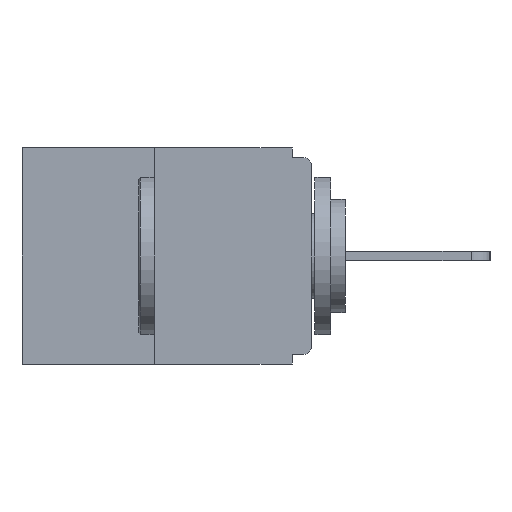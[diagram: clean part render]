
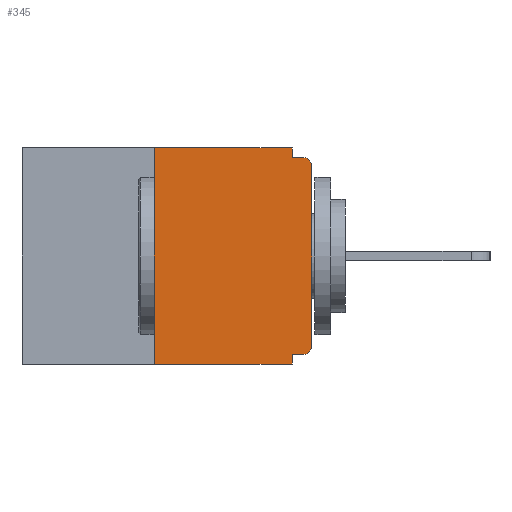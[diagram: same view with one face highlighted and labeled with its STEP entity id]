
A CAD part, left-side view. The second image highlights one B-rep face of the part: STEP entity #345.
In plain terms, the highlighted planar face has unit normal (-1, 0, 0).
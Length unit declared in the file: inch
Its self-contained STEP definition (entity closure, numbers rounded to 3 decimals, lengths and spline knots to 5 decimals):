
#185 = DIRECTION ( 'NONE',  ( -1., 0., 0. ) ) ;
#345 = ADVANCED_FACE ( 'NONE', ( #2129 ), #19526, .F. ) ;
#494 = VECTOR ( 'NONE', #15554, 39.37008 ) ;
#844 = DIRECTION ( 'NONE',  ( 0., 0., -1. ) ) ;
#1202 = ORIENTED_EDGE ( 'NONE', *, *, #11485, .F. ) ;
#1237 = CIRCLE ( 'NONE', #6461, 0.015 ) ;
#1445 = EDGE_CURVE ( 'NONE', #11963, #7149, #10571, .T. ) ;
#1454 = CIRCLE ( 'NONE', #1816, 0.015 ) ;
#1697 = CARTESIAN_POINT ( 'NONE',  ( 0., 0.015, -0.015 ) ) ;
#1816 = AXIS2_PLACEMENT_3D ( 'NONE', #4488, #185, #16967 ) ;
#1875 = CARTESIAN_POINT ( 'NONE',  ( 0., 0.25, 0. ) ) ;
#2006 = VECTOR ( 'NONE', #2769, 39.37008 ) ;
#2129 = FACE_OUTER_BOUND ( 'NONE', #8937, .T. ) ;
#2533 = VECTOR ( 'NONE', #11294, 39.37008 ) ;
#2769 = DIRECTION ( 'NONE',  ( 0., -1., 0. ) ) ;
#3111 = AXIS2_PLACEMENT_3D ( 'NONE', #14575, #17868, #8278 ) ;
#3160 = VECTOR ( 'NONE', #8622, 39.37008 ) ;
#3869 = DIRECTION ( 'NONE',  ( 0., -1., 0. ) ) ;
#3902 = VERTEX_POINT ( 'NONE', #8051 ) ;
#3907 = LINE ( 'NONE', #19870, #3160 ) ;
#3956 = ORIENTED_EDGE ( 'NONE', *, *, #17641, .F. ) ;
#4488 = CARTESIAN_POINT ( 'NONE',  ( 0., 0.015, -0.03 ) ) ;
#4532 = EDGE_CURVE ( 'NONE', #10491, #7149, #1454, .T. ) ;
#4659 = VECTOR ( 'NONE', #15467, 39.37008 ) ;
#4820 = EDGE_CURVE ( 'NONE', #3902, #16959, #5487, .T. ) ;
#4845 = ORIENTED_EDGE ( 'NONE', *, *, #18654, .F. ) ;
#5487 = LINE ( 'NONE', #10337, #8335 ) ;
#5598 = ORIENTED_EDGE ( 'NONE', *, *, #19945, .T. ) ;
#5983 = ORIENTED_EDGE ( 'NONE', *, *, #17176, .F. ) ;
#6461 = AXIS2_PLACEMENT_3D ( 'NONE', #16472, #16691, #844 ) ;
#6522 = LINE ( 'NONE', #12842, #2533 ) ;
#6594 = LINE ( 'NONE', #6694, #9418 ) ;
#6694 = CARTESIAN_POINT ( 'NONE',  ( 0., 0.46, 0. ) ) ;
#7149 = VERTEX_POINT ( 'NONE', #1697 ) ;
#7938 = CARTESIAN_POINT ( 'NONE',  ( 0., 0., -0.313 ) ) ;
#8051 = CARTESIAN_POINT ( 'NONE',  ( 0., 0.25, -0.343 ) ) ;
#8278 = DIRECTION ( 'NONE',  ( 0., 0., -1. ) ) ;
#8335 = VECTOR ( 'NONE', #3869, 39.37008 ) ;
#8622 = DIRECTION ( 'NONE',  ( 0., 0., -1. ) ) ;
#8937 = EDGE_LOOP ( 'NONE', ( #3956, #15534, #14204, #1202, #5983, #5598, #11415, #13940, #19472, #4845 ) ) ;
#9338 = EDGE_CURVE ( 'NONE', #17941, #10491, #11219, .T. ) ;
#9418 = VECTOR ( 'NONE', #19209, 39.37008 ) ;
#9718 = CARTESIAN_POINT ( 'NONE',  ( 0., 0.031, 0. ) ) ;
#9989 = CARTESIAN_POINT ( 'NONE',  ( 0., 0.031, -0.328 ) ) ;
#10284 = CARTESIAN_POINT ( 'NONE',  ( 0., 0.25, 0. ) ) ;
#10337 = CARTESIAN_POINT ( 'NONE',  ( 0., 0.46, -0.343 ) ) ;
#10476 = CARTESIAN_POINT ( 'NONE',  ( 0., 0., -0.015 ) ) ;
#10491 = VERTEX_POINT ( 'NONE', #11611 ) ;
#10571 = LINE ( 'NONE', #10476, #2006 ) ;
#10915 = CARTESIAN_POINT ( 'NONE',  ( 0., 0., 0. ) ) ;
#11046 = VECTOR ( 'NONE', #18880, 39.37008 ) ;
#11219 = LINE ( 'NONE', #10915, #494 ) ;
#11294 = DIRECTION ( 'NONE',  ( 0., 1., 0. ) ) ;
#11400 = CARTESIAN_POINT ( 'NONE',  ( 0., 0.015, -0.328 ) ) ;
#11415 = ORIENTED_EDGE ( 'NONE', *, *, #9338, .T. ) ;
#11485 = EDGE_CURVE ( 'NONE', #18072, #16959, #12284, .T. ) ;
#11611 = CARTESIAN_POINT ( 'NONE',  ( 0., 0., -0.03 ) ) ;
#11963 = VERTEX_POINT ( 'NONE', #15140 ) ;
#12284 = LINE ( 'NONE', #18460, #4659 ) ;
#12842 = CARTESIAN_POINT ( 'NONE',  ( 0., 0., -0.328 ) ) ;
#13940 = ORIENTED_EDGE ( 'NONE', *, *, #4532, .T. ) ;
#13950 = VERTEX_POINT ( 'NONE', #10284 ) ;
#14204 = ORIENTED_EDGE ( 'NONE', *, *, #4820, .T. ) ;
#14575 = CARTESIAN_POINT ( 'NONE',  ( 0., 0.46, 0. ) ) ;
#14825 = VERTEX_POINT ( 'NONE', #9718 ) ;
#15140 = CARTESIAN_POINT ( 'NONE',  ( 0., 0.031, -0.015 ) ) ;
#15467 = DIRECTION ( 'NONE',  ( 0., 0., -1. ) ) ;
#15534 = ORIENTED_EDGE ( 'NONE', *, *, #16710, .F. ) ;
#15554 = DIRECTION ( 'NONE',  ( 0., 0., 1. ) ) ;
#15970 = LINE ( 'NONE', #1875, #11046 ) ;
#16472 = CARTESIAN_POINT ( 'NONE',  ( 0., 0.015, -0.313 ) ) ;
#16691 = DIRECTION ( 'NONE',  ( -1., 0., 0. ) ) ;
#16710 = EDGE_CURVE ( 'NONE', #3902, #13950, #15970, .T. ) ;
#16959 = VERTEX_POINT ( 'NONE', #18934 ) ;
#16967 = DIRECTION ( 'NONE',  ( 0., 0., -1. ) ) ;
#17087 = VERTEX_POINT ( 'NONE', #11400 ) ;
#17176 = EDGE_CURVE ( 'NONE', #17087, #18072, #6522, .T. ) ;
#17641 = EDGE_CURVE ( 'NONE', #13950, #14825, #6594, .T. ) ;
#17868 = DIRECTION ( 'NONE',  ( 1., 0., 0. ) ) ;
#17941 = VERTEX_POINT ( 'NONE', #7938 ) ;
#18072 = VERTEX_POINT ( 'NONE', #9989 ) ;
#18460 = CARTESIAN_POINT ( 'NONE',  ( 0., 0.031, -0.343 ) ) ;
#18654 = EDGE_CURVE ( 'NONE', #14825, #11963, #3907, .T. ) ;
#18880 = DIRECTION ( 'NONE',  ( 0., 0., 1. ) ) ;
#18934 = CARTESIAN_POINT ( 'NONE',  ( 0., 0.031, -0.343 ) ) ;
#19209 = DIRECTION ( 'NONE',  ( 0., -1., 0. ) ) ;
#19472 = ORIENTED_EDGE ( 'NONE', *, *, #1445, .F. ) ;
#19526 = PLANE ( 'NONE',  #3111 ) ;
#19870 = CARTESIAN_POINT ( 'NONE',  ( 0., 0.031, 0. ) ) ;
#19945 = EDGE_CURVE ( 'NONE', #17087, #17941, #1237, .T. ) ;
